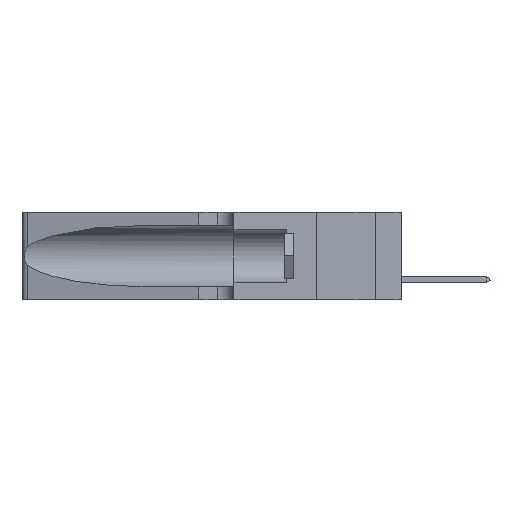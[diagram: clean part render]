
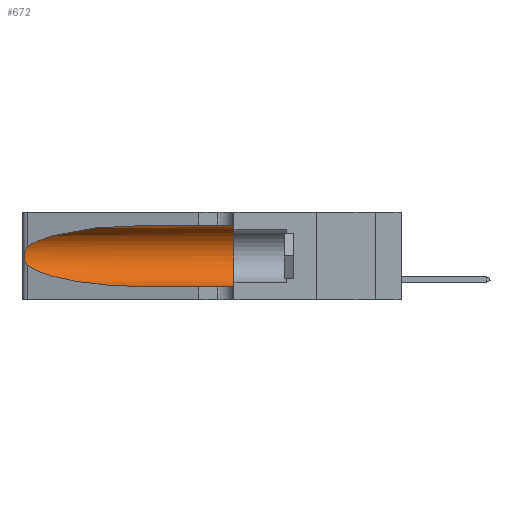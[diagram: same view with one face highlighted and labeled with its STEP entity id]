
A CAD part, left-side view. The second image highlights one B-rep face of the part: STEP entity #672.
In plain terms, the highlighted cylindrical face has radius 3.308 mm (diameter 6.617 mm), a partial arc.
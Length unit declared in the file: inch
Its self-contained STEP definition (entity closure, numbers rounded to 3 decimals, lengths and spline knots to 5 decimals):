
#106 = VECTOR ( 'NONE', #16427, 39.37008 ) ;
#338 = CARTESIAN_POINT ( 'NONE',  ( 0.25639, 1.23184, 0.21858 ) ) ;
#626 = CARTESIAN_POINT ( 'NONE',  ( 0.1305, 0.35, 0.31525 ) ) ;
#672 = ADVANCED_FACE ( 'NONE', ( #38872 ), #14152, .F. ) ;
#1465 = ORIENTED_EDGE ( 'NONE', *, *, #23102, .T. ) ;
#2712 = DIRECTION ( 'NONE',  ( 0., 0., 1. ) ) ;
#2764 = VERTEX_POINT ( 'NONE', #8984 ) ;
#3810 = DIRECTION ( 'NONE',  ( 0., -1., 0. ) ) ;
#6434 = VECTOR ( 'NONE', #32016, 39.37008 ) ;
#6455 = CARTESIAN_POINT ( 'NONE',  ( 0.25787, 1.23484, 0.2124 ) ) ;
#7111 = CARTESIAN_POINT ( 'NONE',  ( 0.1305, 1.61858, 0.31525 ) ) ;
#7913 = CARTESIAN_POINT ( 'NONE',  ( 0.25487, 1.22718, 0.22369 ) ) ;
#8185 = EDGE_CURVE ( 'NONE', #19723, #37192, #16981, .T. ) ;
#8198 = VERTEX_POINT ( 'NONE', #7913 ) ;
#8984 = CARTESIAN_POINT ( 'NONE',  ( 0.1305, 0.72297, 0.31525 ) ) ;
#9112 = CARTESIAN_POINT ( 'NONE',  ( 0.18966, 0.96281, 0.31525 ) ) ;
#9118 = CIRCLE ( 'NONE', #27533, 0.13025 ) ;
#9218 = CARTESIAN_POINT ( 'NONE',  ( 0.25854, 1.2359, 0.20912 ) ) ;
#10323 = EDGE_LOOP ( 'NONE', ( #22332, #1465, #16579, #27743, #32886, #18958 ) ) ;
#10377 = CARTESIAN_POINT ( 'NONE',  ( 0.1305, 1.61858, 0.05475 ) ) ;
#10744 = CARTESIAN_POINT ( 'NONE',  ( 0.2373, 1.15595, 0.08982 ) ) ;
#10887 = CARTESIAN_POINT ( 'NONE',  ( 0.18966, 0.96281, 0.05475 ) ) ;
#11527 = EDGE_CURVE ( 'NONE', #18014, #39254, #9118, .T. ) ;
#11662 = AXIS2_PLACEMENT_3D ( 'NONE', #21592, #3810, #15873 ) ;
#12458 = CARTESIAN_POINT ( 'NONE',  ( 0.26017, 1.23833, 0.17102 ) ) ;
#13399 = EDGE_CURVE ( 'NONE', #37192, #39254, #14682, .T. ) ;
#13517 = B_SPLINE_CURVE_WITH_KNOTS ( 'NONE', 3,
 ( #15776, #18535, #338, #6455, #9218, #37188, #30979, #37451, #12458, #18910, #30837, #34060, #31104, #15536 ),
 .UNSPECIFIED., .F., .F.,
 ( 4, 2, 2, 2, 2, 2, 4 ),
 ( 0., 0.00027, 0.00053, 0.00107, 0.0016, 0.00187, 0.00214 ),
 .UNSPECIFIED. ) ;
#14152 = CYLINDRICAL_SURFACE ( 'NONE', #11662, 0.13025 ) ;
#14682 = LINE ( 'NONE', #10377, #6434 ) ;
#15536 = CARTESIAN_POINT ( 'NONE',  ( 0.25487, 1.22718, 0.14631 ) ) ;
#15776 = CARTESIAN_POINT ( 'NONE',  ( 0.25487, 1.22718, 0.22369 ) ) ;
#15804 = CARTESIAN_POINT ( 'NONE',  ( 0.25487, 1.22718, 0.22369 ) ) ;
#15873 = DIRECTION ( 'NONE',  ( 0., 0., -1. ) ) ;
#16427 = DIRECTION ( 'NONE',  ( 0., -1., 0. ) ) ;
#16579 = ORIENTED_EDGE ( 'NONE', *, *, #8185, .T. ) ;
#16981 =( BOUNDED_CURVE ( )  B_SPLINE_CURVE ( 3, ( #23459, #10744, #10887, #38503 ),
 .UNSPECIFIED., .F., .T. ) 
 B_SPLINE_CURVE_WITH_KNOTS ( ( 4, 4 ),
 ( 3.44316, 4.71239 ),
 .UNSPECIFIED. ) 
 CURVE ( )  GEOMETRIC_REPRESENTATION_ITEM ( )  RATIONAL_B_SPLINE_CURVE ( ( 1., 0.87, 0.87, 1. ) ) 
 REPRESENTATION_ITEM ( '' )  );
#18014 = VERTEX_POINT ( 'NONE', #626 ) ;
#18056 = DIRECTION ( 'NONE',  ( 0., 1., 0. ) ) ;
#18535 = CARTESIAN_POINT ( 'NONE',  ( 0.25555, 1.22994, 0.2215 ) ) ;
#18910 = CARTESIAN_POINT ( 'NONE',  ( 0.25856, 1.23593, 0.16098 ) ) ;
#18958 = ORIENTED_EDGE ( 'NONE', *, *, #23224, .F. ) ;
#19723 = VERTEX_POINT ( 'NONE', #27196 ) ;
#21592 = CARTESIAN_POINT ( 'NONE',  ( 0.1305, 1.61858, 0.185 ) ) ;
#22332 = ORIENTED_EDGE ( 'NONE', *, *, #27752, .T. ) ;
#23102 = EDGE_CURVE ( 'NONE', #8198, #19723, #13517, .T. ) ;
#23172 =( BOUNDED_CURVE ( )  B_SPLINE_CURVE ( 3, ( #27805, #9112, #24915, #15804 ),
 .UNSPECIFIED., .F., .T. ) 
 B_SPLINE_CURVE_WITH_KNOTS ( ( 4, 4 ),
 ( 1.5708, 2.84003 ),
 .UNSPECIFIED. ) 
 CURVE ( )  GEOMETRIC_REPRESENTATION_ITEM ( )  RATIONAL_B_SPLINE_CURVE ( ( 1., 0.87, 0.87, 1. ) ) 
 REPRESENTATION_ITEM ( '' )  );
#23224 = EDGE_CURVE ( 'NONE', #2764, #18014, #34925, .T. ) ;
#23459 = CARTESIAN_POINT ( 'NONE',  ( 0.25487, 1.22718, 0.14631 ) ) ;
#24915 = CARTESIAN_POINT ( 'NONE',  ( 0.2373, 1.15595, 0.28018 ) ) ;
#26233 = CARTESIAN_POINT ( 'NONE',  ( 0.1305, 0.35, 0.05475 ) ) ;
#27196 = CARTESIAN_POINT ( 'NONE',  ( 0.25487, 1.22718, 0.14631 ) ) ;
#27533 = AXIS2_PLACEMENT_3D ( 'NONE', #33972, #18056, #2712 ) ;
#27743 = ORIENTED_EDGE ( 'NONE', *, *, #13399, .T. ) ;
#27752 = EDGE_CURVE ( 'NONE', #2764, #8198, #23172, .T. ) ;
#27805 = CARTESIAN_POINT ( 'NONE',  ( 0.1305, 0.72297, 0.31525 ) ) ;
#30837 = CARTESIAN_POINT ( 'NONE',  ( 0.25789, 1.23486, 0.15765 ) ) ;
#30979 = CARTESIAN_POINT ( 'NONE',  ( 0.26075, 1.23896, 0.19203 ) ) ;
#31009 = CARTESIAN_POINT ( 'NONE',  ( 0.1305, 0.72297, 0.05475 ) ) ;
#31104 = CARTESIAN_POINT ( 'NONE',  ( 0.25555, 1.22993, 0.14849 ) ) ;
#32016 = DIRECTION ( 'NONE',  ( 0., -1., 0. ) ) ;
#32886 = ORIENTED_EDGE ( 'NONE', *, *, #11527, .F. ) ;
#33972 = CARTESIAN_POINT ( 'NONE',  ( 0.1305, 0.35, 0.185 ) ) ;
#34060 = CARTESIAN_POINT ( 'NONE',  ( 0.25639, 1.23186, 0.15144 ) ) ;
#34925 = LINE ( 'NONE', #7111, #106 ) ;
#37188 = CARTESIAN_POINT ( 'NONE',  ( 0.26018, 1.23835, 0.19895 ) ) ;
#37192 = VERTEX_POINT ( 'NONE', #31009 ) ;
#37451 = CARTESIAN_POINT ( 'NONE',  ( 0.26075, 1.23896, 0.178 ) ) ;
#38503 = CARTESIAN_POINT ( 'NONE',  ( 0.1305, 0.72297, 0.05475 ) ) ;
#38872 = FACE_OUTER_BOUND ( 'NONE', #10323, .T. ) ;
#39254 = VERTEX_POINT ( 'NONE', #26233 ) ;
